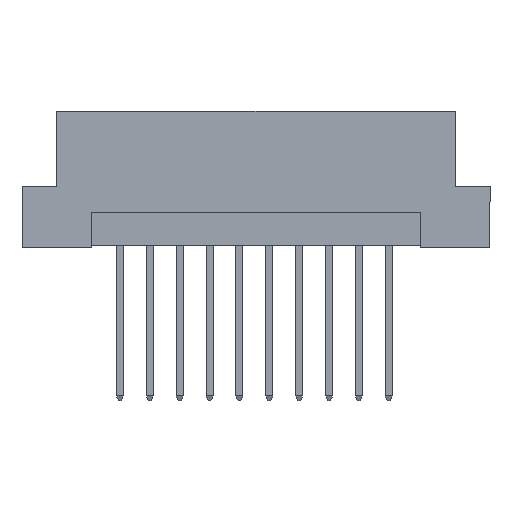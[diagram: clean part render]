
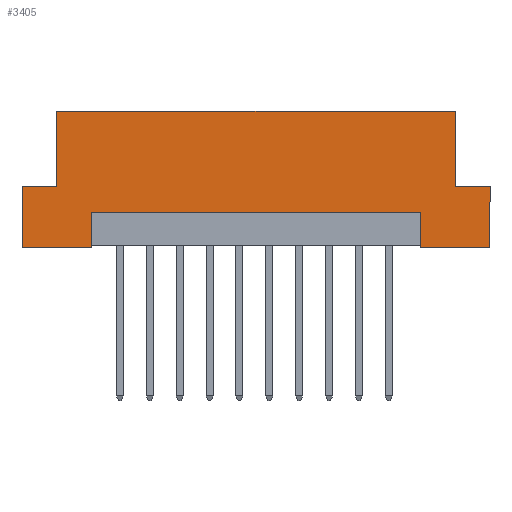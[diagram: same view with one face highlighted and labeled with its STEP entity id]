
A CAD part, front view. The second image highlights one B-rep face of the part: STEP entity #3405.
In plain terms, the highlighted planar face has unit normal (0, -1, 0).
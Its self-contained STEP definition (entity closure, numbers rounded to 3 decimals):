
#27 = AXIS2_PLACEMENT_3D ( 'NONE', #906, #2577, #4705 ) ;
#98 = VERTEX_POINT ( 'NONE', #2216 ) ;
#150 = DIRECTION ( 'NONE',  ( 0., 0., 1. ) ) ;
#155 = CARTESIAN_POINT ( 'NONE',  ( -19.9, -4.3, 5.2 ) ) ;
#221 = EDGE_CURVE ( 'NONE', #4299, #98, #2874, .T. ) ;
#318 = CARTESIAN_POINT ( 'NONE',  ( 16.94, -4.3, 11.6 ) ) ;
#376 = CARTESIAN_POINT ( 'NONE',  ( -14., -4.3, 0.2 ) ) ;
#417 = LINE ( 'NONE', #4212, #3471 ) ;
#430 = VERTEX_POINT ( 'NONE', #3505 ) ;
#480 = VECTOR ( 'NONE', #2280, 1000. ) ;
#552 = ORIENTED_EDGE ( 'NONE', *, *, #2249, .F. ) ;
#581 = LINE ( 'NONE', #155, #4345 ) ;
#650 = EDGE_CURVE ( 'NONE', #430, #98, #2936, .T. ) ;
#707 = ORIENTED_EDGE ( 'NONE', *, *, #2574, .F. ) ;
#723 = VERTEX_POINT ( 'NONE', #4340 ) ;
#743 = EDGE_CURVE ( 'NONE', #3785, #4178, #4427, .T. ) ;
#767 = CARTESIAN_POINT ( 'NONE',  ( -16.94, -4.3, 5.2 ) ) ;
#783 = DIRECTION ( 'NONE',  ( 1., 0., 0. ) ) ;
#796 = DIRECTION ( 'NONE',  ( 0., 0., -1. ) ) ;
#823 = EDGE_CURVE ( 'NONE', #5078, #430, #3750, .T. ) ;
#835 = DIRECTION ( 'NONE',  ( 1., 0., 0. ) ) ;
#887 = CARTESIAN_POINT ( 'NONE',  ( 14., -4.3, 3. ) ) ;
#906 = CARTESIAN_POINT ( 'NONE',  ( 19.9, -4.3, 11.6 ) ) ;
#942 = DIRECTION ( 'NONE',  ( 1., 0., 0. ) ) ;
#986 = ORIENTED_EDGE ( 'NONE', *, *, #2307, .T. ) ;
#1019 = CARTESIAN_POINT ( 'NONE',  ( 14., -4.3, 0.2 ) ) ;
#1125 = VERTEX_POINT ( 'NONE', #767 ) ;
#1211 = LINE ( 'NONE', #4566, #3452 ) ;
#1293 = VERTEX_POINT ( 'NONE', #2234 ) ;
#1385 = DIRECTION ( 'NONE',  ( 1., 0., 0. ) ) ;
#1492 = CARTESIAN_POINT ( 'NONE',  ( 16.94, -4.3, 5.2 ) ) ;
#1870 = VECTOR ( 'NONE', #3638, 1000. ) ;
#1982 = DIRECTION ( 'NONE',  ( 1., 0., 0. ) ) ;
#2005 = LINE ( 'NONE', #2446, #1870 ) ;
#2028 = CARTESIAN_POINT ( 'NONE',  ( -19.9, -4.3, 11.6 ) ) ;
#2216 = CARTESIAN_POINT ( 'NONE',  ( -14., -4.3, 0. ) ) ;
#2225 = ORIENTED_EDGE ( 'NONE', *, *, #2246, .T. ) ;
#2234 = CARTESIAN_POINT ( 'NONE',  ( 19.9, -4.3, 0. ) ) ;
#2246 = EDGE_CURVE ( 'NONE', #3360, #1293, #5356, .T. ) ;
#2249 = EDGE_CURVE ( 'NONE', #5073, #4178, #4594, .T. ) ;
#2251 = DIRECTION ( 'NONE',  ( 0., 0., 1. ) ) ;
#2280 = DIRECTION ( 'NONE',  ( 0., 0., 1. ) ) ;
#2307 = EDGE_CURVE ( 'NONE', #4299, #4547, #417, .T. ) ;
#2420 = CARTESIAN_POINT ( 'NONE',  ( 19.9, -4.3, 11.6 ) ) ;
#2446 = CARTESIAN_POINT ( 'NONE',  ( 19.9, -4.3, 5.2 ) ) ;
#2525 = CARTESIAN_POINT ( 'NONE',  ( 19.9, -4.3, 0. ) ) ;
#2574 = EDGE_CURVE ( 'NONE', #5078, #1125, #581, .T. ) ;
#2577 = DIRECTION ( 'NONE',  ( 0., 1., 0. ) ) ;
#2658 = CARTESIAN_POINT ( 'NONE',  ( -16.94, -4.3, 11.6 ) ) ;
#2666 = LINE ( 'NONE', #2721, #480 ) ;
#2671 = ORIENTED_EDGE ( 'NONE', *, *, #743, .T. ) ;
#2721 = CARTESIAN_POINT ( 'NONE',  ( -16.94, -4.3, 5.2 ) ) ;
#2799 = DIRECTION ( 'NONE',  ( 0., 0., -1. ) ) ;
#2874 = LINE ( 'NONE', #376, #4883 ) ;
#2908 = CARTESIAN_POINT ( 'NONE',  ( 19.9, -4.3, 0. ) ) ;
#2936 = LINE ( 'NONE', #2525, #5337 ) ;
#2988 = FACE_OUTER_BOUND ( 'NONE', #3854, .T. ) ;
#3038 = LINE ( 'NONE', #1019, #3278 ) ;
#3150 = ORIENTED_EDGE ( 'NONE', *, *, #221, .F. ) ;
#3152 = CARTESIAN_POINT ( 'NONE',  ( -14., -4.3, 3. ) ) ;
#3278 = VECTOR ( 'NONE', #150, 1000. ) ;
#3295 = VECTOR ( 'NONE', #835, 1000. ) ;
#3328 = CARTESIAN_POINT ( 'NONE',  ( 14., -4.3, 0. ) ) ;
#3360 = VERTEX_POINT ( 'NONE', #3328 ) ;
#3405 = ADVANCED_FACE ( 'NONE', ( #2988 ), #4675, .F. ) ;
#3452 = VECTOR ( 'NONE', #796, 1000. ) ;
#3471 = VECTOR ( 'NONE', #1982, 1000. ) ;
#3505 = CARTESIAN_POINT ( 'NONE',  ( -19.9, -4.3, 0. ) ) ;
#3638 = DIRECTION ( 'NONE',  ( 1., 0., 0. ) ) ;
#3657 = ORIENTED_EDGE ( 'NONE', *, *, #823, .T. ) ;
#3688 = CARTESIAN_POINT ( 'NONE',  ( -19.9, -4.3, 5.2 ) ) ;
#3750 = LINE ( 'NONE', #2028, #5228 ) ;
#3785 = VERTEX_POINT ( 'NONE', #5346 ) ;
#3854 = EDGE_LOOP ( 'NONE', ( #986, #4870, #2225, #4242, #3990, #2671, #552, #4752, #707, #3657, #4929, #3150 ) ) ;
#3968 = EDGE_CURVE ( 'NONE', #723, #1293, #1211, .T. ) ;
#3990 = ORIENTED_EDGE ( 'NONE', *, *, #4804, .F. ) ;
#4133 = EDGE_CURVE ( 'NONE', #3360, #4547, #3038, .T. ) ;
#4170 = VECTOR ( 'NONE', #783, 1000. ) ;
#4178 = VERTEX_POINT ( 'NONE', #318 ) ;
#4212 = CARTESIAN_POINT ( 'NONE',  ( -14., -4.3, 3. ) ) ;
#4242 = ORIENTED_EDGE ( 'NONE', *, *, #3968, .F. ) ;
#4299 = VERTEX_POINT ( 'NONE', #3152 ) ;
#4340 = CARTESIAN_POINT ( 'NONE',  ( 19.9, -4.3, 5.2 ) ) ;
#4345 = VECTOR ( 'NONE', #1385, 1000. ) ;
#4427 = LINE ( 'NONE', #1492, #5320 ) ;
#4547 = VERTEX_POINT ( 'NONE', #887 ) ;
#4566 = CARTESIAN_POINT ( 'NONE',  ( 19.9, -4.3, 11.6 ) ) ;
#4594 = LINE ( 'NONE', #2420, #4170 ) ;
#4597 = EDGE_CURVE ( 'NONE', #1125, #5073, #2666, .T. ) ;
#4675 = PLANE ( 'NONE',  #27 ) ;
#4705 = DIRECTION ( 'NONE',  ( -1., 0., 0. ) ) ;
#4752 = ORIENTED_EDGE ( 'NONE', *, *, #4597, .F. ) ;
#4804 = EDGE_CURVE ( 'NONE', #3785, #723, #2005, .T. ) ;
#4870 = ORIENTED_EDGE ( 'NONE', *, *, #4133, .F. ) ;
#4883 = VECTOR ( 'NONE', #5420, 1000. ) ;
#4929 = ORIENTED_EDGE ( 'NONE', *, *, #650, .T. ) ;
#5073 = VERTEX_POINT ( 'NONE', #2658 ) ;
#5078 = VERTEX_POINT ( 'NONE', #3688 ) ;
#5228 = VECTOR ( 'NONE', #2799, 1000. ) ;
#5320 = VECTOR ( 'NONE', #2251, 1000. ) ;
#5337 = VECTOR ( 'NONE', #942, 1000. ) ;
#5346 = CARTESIAN_POINT ( 'NONE',  ( 16.94, -4.3, 5.2 ) ) ;
#5356 = LINE ( 'NONE', #2908, #3295 ) ;
#5420 = DIRECTION ( 'NONE',  ( 0., 0., -1. ) ) ;
